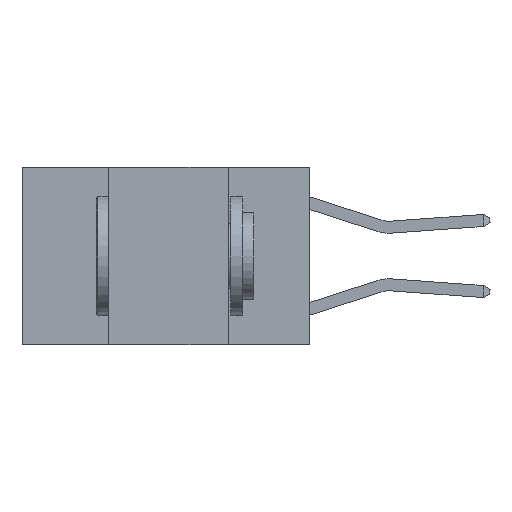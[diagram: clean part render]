
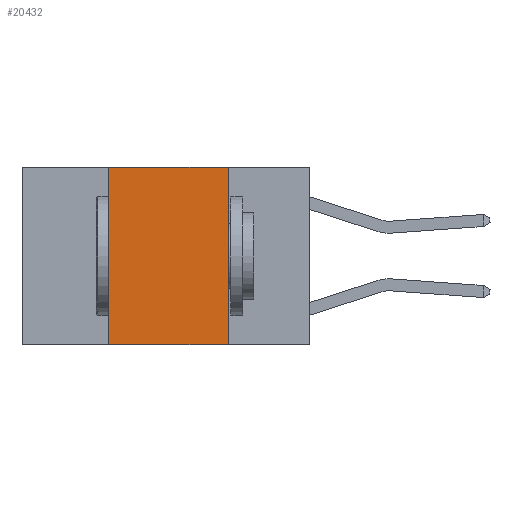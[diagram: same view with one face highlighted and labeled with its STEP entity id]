
A CAD part, left-side view. The second image highlights one B-rep face of the part: STEP entity #20432.
In plain terms, the highlighted planar face has unit normal (-1, 0, 0).
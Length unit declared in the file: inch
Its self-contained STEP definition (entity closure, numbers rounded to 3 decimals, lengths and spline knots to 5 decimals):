
#750 = DIRECTION ( 'NONE',  ( 0., -1., 0. ) ) ;
#1114 = LINE ( 'NONE', #11285, #20952 ) ;
#1121 = EDGE_LOOP ( 'NONE', ( #5029, #13102, #19763, #19380 ) ) ;
#1736 = FACE_OUTER_BOUND ( 'NONE', #1121, .T. ) ;
#1783 = LINE ( 'NONE', #3954, #9651 ) ;
#2927 = CARTESIAN_POINT ( 'NONE',  ( 0., 0.42, -0.37 ) ) ;
#3832 = DIRECTION ( 'NONE',  ( 0., -1., 0. ) ) ;
#3954 = CARTESIAN_POINT ( 'NONE',  ( 0., 0.6, -0.37 ) ) ;
#4710 = VERTEX_POINT ( 'NONE', #5937 ) ;
#5029 = ORIENTED_EDGE ( 'NONE', *, *, #8400, .F. ) ;
#5937 = CARTESIAN_POINT ( 'NONE',  ( 0., 0.17, -0.37 ) ) ;
#6045 = DIRECTION ( 'NONE',  ( 0., 0., -1. ) ) ;
#8400 = EDGE_CURVE ( 'NONE', #11944, #4710, #21436, .T. ) ;
#8984 = EDGE_CURVE ( 'NONE', #19839, #17121, #1114, .T. ) ;
#9651 = VECTOR ( 'NONE', #750, 39.37008 ) ;
#10698 = EDGE_CURVE ( 'NONE', #17121, #11944, #16264, .T. ) ;
#10857 = VECTOR ( 'NONE', #3832, 39.37008 ) ;
#11285 = CARTESIAN_POINT ( 'NONE',  ( 0., 0.42, 0. ) ) ;
#11944 = VERTEX_POINT ( 'NONE', #16987 ) ;
#12539 = CARTESIAN_POINT ( 'NONE',  ( 0., 0.17, 0. ) ) ;
#12944 = CARTESIAN_POINT ( 'NONE',  ( 0., 0.6, 0. ) ) ;
#13102 = ORIENTED_EDGE ( 'NONE', *, *, #10698, .F. ) ;
#13707 = PLANE ( 'NONE',  #13741 ) ;
#13741 = AXIS2_PLACEMENT_3D ( 'NONE', #18830, #15646, #17013 ) ;
#15021 = DIRECTION ( 'NONE',  ( 0., 0., 1. ) ) ;
#15552 = EDGE_CURVE ( 'NONE', #19839, #4710, #1783, .T. ) ;
#15646 = DIRECTION ( 'NONE',  ( 1., 0., 0. ) ) ;
#16264 = LINE ( 'NONE', #12944, #10857 ) ;
#16987 = CARTESIAN_POINT ( 'NONE',  ( 0., 0.17, 0. ) ) ;
#17013 = DIRECTION ( 'NONE',  ( 0., 0., -1. ) ) ;
#17121 = VERTEX_POINT ( 'NONE', #21919 ) ;
#18830 = CARTESIAN_POINT ( 'NONE',  ( 0., 0.6, 0. ) ) ;
#19380 = ORIENTED_EDGE ( 'NONE', *, *, #15552, .T. ) ;
#19763 = ORIENTED_EDGE ( 'NONE', *, *, #8984, .F. ) ;
#19839 = VERTEX_POINT ( 'NONE', #2927 ) ;
#20432 = ADVANCED_FACE ( 'NONE', ( #1736 ), #13707, .F. ) ;
#20918 = VECTOR ( 'NONE', #6045, 39.37008 ) ;
#20952 = VECTOR ( 'NONE', #15021, 39.37008 ) ;
#21436 = LINE ( 'NONE', #12539, #20918 ) ;
#21919 = CARTESIAN_POINT ( 'NONE',  ( 0., 0.42, 0. ) ) ;
